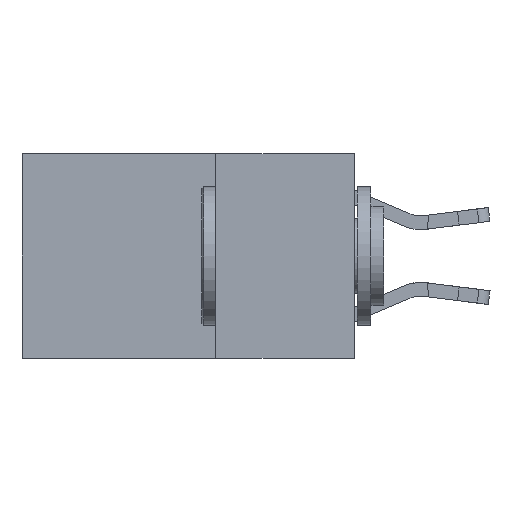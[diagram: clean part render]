
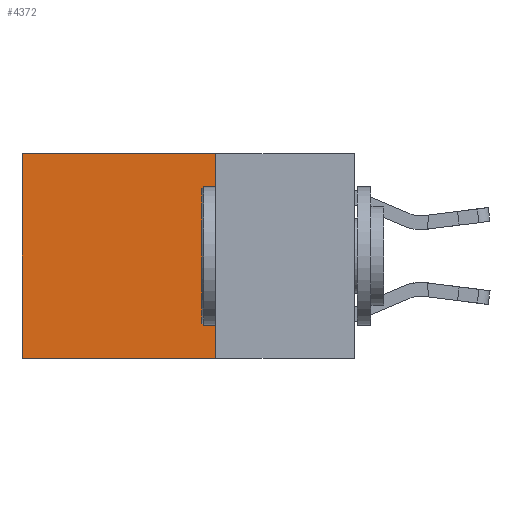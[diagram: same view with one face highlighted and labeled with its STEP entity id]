
A CAD part, left-side view. The second image highlights one B-rep face of the part: STEP entity #4372.
In plain terms, the highlighted planar face has unit normal (-1, 0, 0).
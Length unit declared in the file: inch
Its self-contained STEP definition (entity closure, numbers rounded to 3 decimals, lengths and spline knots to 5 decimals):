
#276 = DIRECTION ( 'NONE',  ( 0., 1., 0. ) ) ;
#832 = CARTESIAN_POINT ( 'NONE',  ( 0.2625, 0.25, 0. ) ) ;
#1189 = CARTESIAN_POINT ( 'NONE',  ( 0.2625, 0.25, 0. ) ) ;
#1277 = LINE ( 'NONE', #1189, #4768 ) ;
#1719 = CARTESIAN_POINT ( 'NONE',  ( 0.2625, 0.25, 0. ) ) ;
#2880 = EDGE_CURVE ( 'NONE', #5676, #10455, #13448, .T. ) ;
#3106 = EDGE_CURVE ( 'NONE', #13547, #5676, #23018, .T. ) ;
#3206 = DIRECTION ( 'NONE',  ( 0., 1., 0. ) ) ;
#4372 = ADVANCED_FACE ( 'NONE', ( #19985 ), #21727, .F. ) ;
#4768 = VECTOR ( 'NONE', #3206, 39.37008 ) ;
#5279 = ORIENTED_EDGE ( 'NONE', *, *, #14935, .T. ) ;
#5676 = VERTEX_POINT ( 'NONE', #11577 ) ;
#6969 = CARTESIAN_POINT ( 'NONE',  ( 0.2625, 0.25, 0. ) ) ;
#9556 = EDGE_CURVE ( 'NONE', #13547, #13839, #1277, .T. ) ;
#9846 = DIRECTION ( 'NONE',  ( 1., 0., 0. ) ) ;
#10318 = CARTESIAN_POINT ( 'NONE',  ( 0.2625, 0.25, -0.37 ) ) ;
#10455 = VERTEX_POINT ( 'NONE', #18686 ) ;
#11303 = VECTOR ( 'NONE', #14806, 39.37008 ) ;
#11577 = CARTESIAN_POINT ( 'NONE',  ( 0.2625, 0.25, -0.37 ) ) ;
#13121 = VECTOR ( 'NONE', #20880, 39.37008 ) ;
#13448 = LINE ( 'NONE', #10318, #23357 ) ;
#13547 = VERTEX_POINT ( 'NONE', #832 ) ;
#13839 = VERTEX_POINT ( 'NONE', #19700 ) ;
#14806 = DIRECTION ( 'NONE',  ( 0., 0., -1. ) ) ;
#14935 = EDGE_CURVE ( 'NONE', #13839, #10455, #17870, .T. ) ;
#17400 = EDGE_LOOP ( 'NONE', ( #5279, #20867, #20968, #18563 ) ) ;
#17870 = LINE ( 'NONE', #24840, #11303 ) ;
#18563 = ORIENTED_EDGE ( 'NONE', *, *, #9556, .T. ) ;
#18686 = CARTESIAN_POINT ( 'NONE',  ( 0.2625, 0.6, -0.37 ) ) ;
#19700 = CARTESIAN_POINT ( 'NONE',  ( 0.2625, 0.6, 0. ) ) ;
#19985 = FACE_OUTER_BOUND ( 'NONE', #17400, .T. ) ;
#20867 = ORIENTED_EDGE ( 'NONE', *, *, #2880, .F. ) ;
#20880 = DIRECTION ( 'NONE',  ( 0., 0., -1. ) ) ;
#20968 = ORIENTED_EDGE ( 'NONE', *, *, #3106, .F. ) ;
#21727 = PLANE ( 'NONE',  #25739 ) ;
#23018 = LINE ( 'NONE', #6969, #13121 ) ;
#23357 = VECTOR ( 'NONE', #276, 39.37008 ) ;
#23718 = DIRECTION ( 'NONE',  ( 0., 0., -1. ) ) ;
#24840 = CARTESIAN_POINT ( 'NONE',  ( 0.2625, 0.6, 0. ) ) ;
#25739 = AXIS2_PLACEMENT_3D ( 'NONE', #1719, #9846, #23718 ) ;
